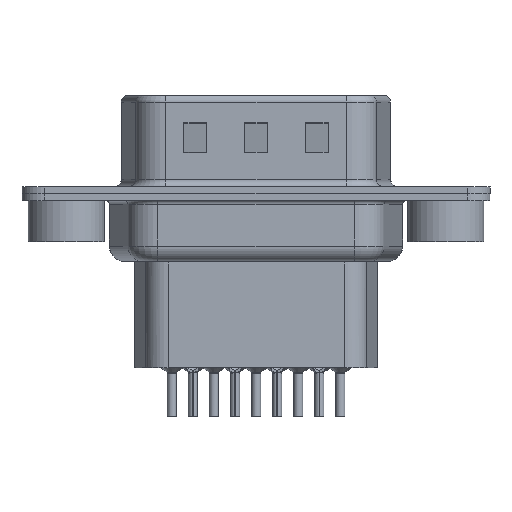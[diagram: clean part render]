
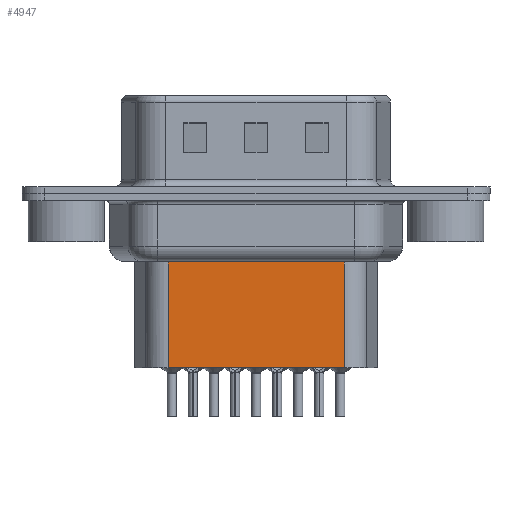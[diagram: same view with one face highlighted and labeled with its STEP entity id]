
A CAD part, front view. The second image highlights one B-rep face of the part: STEP entity #4947.
In plain terms, the highlighted planar face has unit normal (0, -1, 0).
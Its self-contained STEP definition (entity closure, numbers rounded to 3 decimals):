
#45 = CARTESIAN_POINT ( 'NONE',  ( 6.706, -3.5, -11.45 ) ) ;
#659 = LINE ( 'NONE', #18512, #15487 ) ;
#801 = EDGE_CURVE ( 'NONE', #16398, #15313, #13211, .T. ) ;
#1793 = EDGE_CURVE ( 'NONE', #15313, #4835, #11585, .T. ) ;
#2688 = EDGE_CURVE ( 'NONE', #9551, #4835, #14715, .T. ) ;
#3565 = CARTESIAN_POINT ( 'NONE',  ( 6.706, -3.5, -4.097 ) ) ;
#4103 = DIRECTION ( 'NONE',  ( 0., 0., -1. ) ) ;
#4835 = VERTEX_POINT ( 'NONE', #45 ) ;
#4947 = ADVANCED_FACE ( 'NONE', ( #13753 ), #9216, .T. ) ;
#5516 = CARTESIAN_POINT ( 'NONE',  ( 6.706, -3.5, -3.1 ) ) ;
#5629 = VECTOR ( 'NONE', #15958, 1000. ) ;
#6970 = EDGE_CURVE ( 'NONE', #16398, #9551, #659, .T. ) ;
#7063 = ORIENTED_EDGE ( 'NONE', *, *, #6970, .F. ) ;
#7248 = ORIENTED_EDGE ( 'NONE', *, *, #1793, .T. ) ;
#8979 = DIRECTION ( 'NONE',  ( 0., -1., 0. ) ) ;
#9216 = PLANE ( 'NONE',  #11964 ) ;
#9551 = VERTEX_POINT ( 'NONE', #17352 ) ;
#9800 = DIRECTION ( 'NONE',  ( 0., 0., -1. ) ) ;
#10677 = CARTESIAN_POINT ( 'NONE',  ( 6.459, -3.5, -4.097 ) ) ;
#11041 = DIRECTION ( 'NONE',  ( 1., 0., 0. ) ) ;
#11585 = LINE ( 'NONE', #17128, #18437 ) ;
#11834 = EDGE_LOOP ( 'NONE', ( #7063, #12379, #7248, #12442 ) ) ;
#11964 = AXIS2_PLACEMENT_3D ( 'NONE', #5516, #8979, #11041 ) ;
#12379 = ORIENTED_EDGE ( 'NONE', *, *, #801, .T. ) ;
#12442 = ORIENTED_EDGE ( 'NONE', *, *, #2688, .F. ) ;
#13211 = LINE ( 'NONE', #10677, #5629 ) ;
#13753 = FACE_OUTER_BOUND ( 'NONE', #11834, .T. ) ;
#14367 = CARTESIAN_POINT ( 'NONE',  ( 18.294, -3.5, -4.097 ) ) ;
#14505 = CARTESIAN_POINT ( 'NONE',  ( 6.706, -3.5, -11.45 ) ) ;
#14568 = DIRECTION ( 'NONE',  ( -1., 0., 0. ) ) ;
#14715 = LINE ( 'NONE', #14505, #18167 ) ;
#15313 = VERTEX_POINT ( 'NONE', #3565 ) ;
#15487 = VECTOR ( 'NONE', #9800, 1000. ) ;
#15958 = DIRECTION ( 'NONE',  ( -1., 0., 0. ) ) ;
#16398 = VERTEX_POINT ( 'NONE', #14367 ) ;
#17128 = CARTESIAN_POINT ( 'NONE',  ( 6.706, -3.5, -3.1 ) ) ;
#17352 = CARTESIAN_POINT ( 'NONE',  ( 18.294, -3.5, -11.45 ) ) ;
#18167 = VECTOR ( 'NONE', #14568, 1000. ) ;
#18437 = VECTOR ( 'NONE', #4103, 1000. ) ;
#18512 = CARTESIAN_POINT ( 'NONE',  ( 18.294, -3.5, -3.1 ) ) ;
